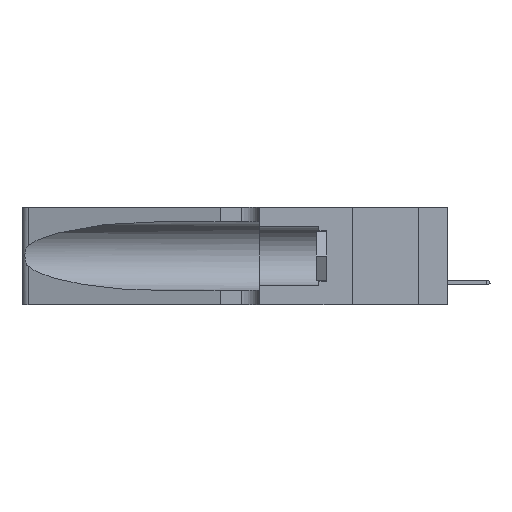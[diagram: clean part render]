
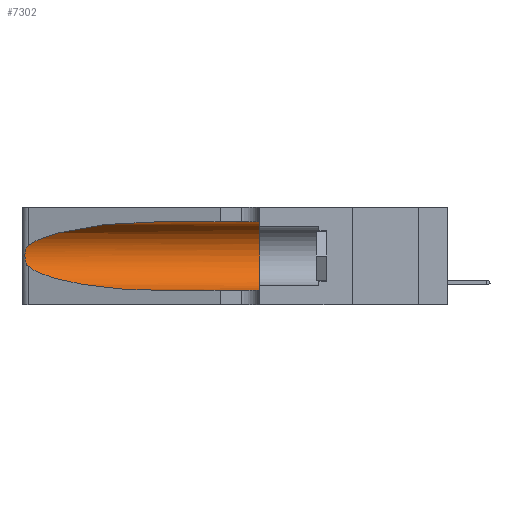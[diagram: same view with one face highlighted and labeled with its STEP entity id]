
A CAD part, left-side view. The second image highlights one B-rep face of the part: STEP entity #7302.
In plain terms, the highlighted cylindrical face has radius 3.308 mm (diameter 6.617 mm), a partial arc.
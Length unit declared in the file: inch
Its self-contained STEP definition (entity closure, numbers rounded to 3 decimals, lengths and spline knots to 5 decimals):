
#775 = CARTESIAN_POINT ( 'NONE',  ( 0.26075, 1.23896, 0.19203 ) ) ;
#2974 = CARTESIAN_POINT ( 'NONE',  ( 0.25639, 1.23184, 0.21858 ) ) ;
#3128 = CARTESIAN_POINT ( 'NONE',  ( 0.25487, 1.22718, 0.22369 ) ) ;
#3421 = CARTESIAN_POINT ( 'NONE',  ( 0.18966, 0.96281, 0.31525 ) ) ;
#3547 = DIRECTION ( 'NONE',  ( 0., 1., 0. ) ) ;
#3717 = CARTESIAN_POINT ( 'NONE',  ( 0.25487, 1.22718, 0.14631 ) ) ;
#3810 = CARTESIAN_POINT ( 'NONE',  ( 0.25487, 1.22718, 0.22369 ) ) ;
#4111 = CARTESIAN_POINT ( 'NONE',  ( 0.2373, 1.15595, 0.08982 ) ) ;
#6169 = CARTESIAN_POINT ( 'NONE',  ( 0.26017, 1.23833, 0.17102 ) ) ;
#6350 = VERTEX_POINT ( 'NONE', #21844 ) ;
#6924 = CARTESIAN_POINT ( 'NONE',  ( 0.25487, 1.22718, 0.14631 ) ) ;
#7302 = ADVANCED_FACE ( 'NONE', ( #29287 ), #10750, .F. ) ;
#8679 = AXIS2_PLACEMENT_3D ( 'NONE', #15345, #21358, #27073 ) ;
#8754 = CARTESIAN_POINT ( 'NONE',  ( 0.25854, 1.2359, 0.20912 ) ) ;
#8937 = EDGE_LOOP ( 'NONE', ( #24188, #16238, #22249, #30770, #29146, #13400 ) ) ;
#9082 = CARTESIAN_POINT ( 'NONE',  ( 0.1305, 0.35, 0.185 ) ) ;
#9935 = VERTEX_POINT ( 'NONE', #6924 ) ;
#10750 = CYLINDRICAL_SURFACE ( 'NONE', #8679, 0.13025 ) ;
#11590 = CARTESIAN_POINT ( 'NONE',  ( 0.25555, 1.22993, 0.14849 ) ) ;
#12124 = VECTOR ( 'NONE', #12397, 39.37008 ) ;
#12397 = DIRECTION ( 'NONE',  ( 0., -1., 0. ) ) ;
#13019 = LINE ( 'NONE', #28895, #12124 ) ;
#13400 = ORIENTED_EDGE ( 'NONE', *, *, #24748, .F. ) ;
#14206 = AXIS2_PLACEMENT_3D ( 'NONE', #9082, #3547, #26107 ) ;
#15270 = CARTESIAN_POINT ( 'NONE',  ( 0.1305, 1.61858, 0.05475 ) ) ;
#15345 = CARTESIAN_POINT ( 'NONE',  ( 0.1305, 1.61858, 0.185 ) ) ;
#15560 = CARTESIAN_POINT ( 'NONE',  ( 0.25487, 1.22718, 0.14631 ) ) ;
#16238 = ORIENTED_EDGE ( 'NONE', *, *, #34376, .T. ) ;
#16996 = CARTESIAN_POINT ( 'NONE',  ( 0.25555, 1.22994, 0.2215 ) ) ;
#17118 = VECTOR ( 'NONE', #34750, 39.37008 ) ;
#17711 = CARTESIAN_POINT ( 'NONE',  ( 0.1305, 0.72297, 0.31525 ) ) ;
#18938 = LINE ( 'NONE', #15270, #17118 ) ;
#19024 = VERTEX_POINT ( 'NONE', #30480 ) ;
#20047 = CARTESIAN_POINT ( 'NONE',  ( 0.25856, 1.23593, 0.16098 ) ) ;
#20294 = CARTESIAN_POINT ( 'NONE',  ( 0.26075, 1.23896, 0.178 ) ) ;
#20326 = EDGE_CURVE ( 'NONE', #29961, #6350, #18938, .T. ) ;
#20816 = CARTESIAN_POINT ( 'NONE',  ( 0.18966, 0.96281, 0.05475 ) ) ;
#21358 = DIRECTION ( 'NONE',  ( 0., -1., 0. ) ) ;
#21844 = CARTESIAN_POINT ( 'NONE',  ( 0.1305, 0.35, 0.05475 ) ) ;
#22249 = ORIENTED_EDGE ( 'NONE', *, *, #34624, .T. ) ;
#22451 = B_SPLINE_CURVE_WITH_KNOTS ( 'NONE', 3,
 ( #22461, #16996, #2974, #25640, #8754, #33553, #775, #20294, #6169, #20047, #31317, #34254, #11590, #3717 ),
 .UNSPECIFIED., .F., .F.,
 ( 4, 2, 2, 2, 2, 2, 4 ),
 ( 0., 0.00027, 0.00053, 0.00107, 0.0016, 0.00187, 0.00214 ),
 .UNSPECIFIED. ) ;
#22461 = CARTESIAN_POINT ( 'NONE',  ( 0.25487, 1.22718, 0.22369 ) ) ;
#23833 = CARTESIAN_POINT ( 'NONE',  ( 0.1305, 0.72297, 0.05475 ) ) ;
#24188 = ORIENTED_EDGE ( 'NONE', *, *, #32831, .T. ) ;
#24748 = EDGE_CURVE ( 'NONE', #26904, #19024, #13019, .T. ) ;
#25640 = CARTESIAN_POINT ( 'NONE',  ( 0.25787, 1.23484, 0.2124 ) ) ;
#26107 = DIRECTION ( 'NONE',  ( 0., 0., 1. ) ) ;
#26265 = CARTESIAN_POINT ( 'NONE',  ( 0.1305, 0.72297, 0.05475 ) ) ;
#26363 = CARTESIAN_POINT ( 'NONE',  ( 0.2373, 1.15595, 0.28018 ) ) ;
#26904 = VERTEX_POINT ( 'NONE', #30628 ) ;
#27073 = DIRECTION ( 'NONE',  ( 0., 0., -1. ) ) ;
#28556 = EDGE_CURVE ( 'NONE', #19024, #6350, #29960, .T. ) ;
#28895 = CARTESIAN_POINT ( 'NONE',  ( 0.1305, 1.61858, 0.31525 ) ) ;
#29146 = ORIENTED_EDGE ( 'NONE', *, *, #28556, .F. ) ;
#29287 = FACE_OUTER_BOUND ( 'NONE', #8937, .T. ) ;
#29960 = CIRCLE ( 'NONE', #14206, 0.13025 ) ;
#29961 = VERTEX_POINT ( 'NONE', #26265 ) ;
#30480 = CARTESIAN_POINT ( 'NONE',  ( 0.1305, 0.35, 0.31525 ) ) ;
#30628 = CARTESIAN_POINT ( 'NONE',  ( 0.1305, 0.72297, 0.31525 ) ) ;
#30770 = ORIENTED_EDGE ( 'NONE', *, *, #20326, .T. ) ;
#31317 = CARTESIAN_POINT ( 'NONE',  ( 0.25789, 1.23486, 0.15765 ) ) ;
#32831 = EDGE_CURVE ( 'NONE', #26904, #33304, #35572, .T. ) ;
#32871 =( BOUNDED_CURVE ( )  B_SPLINE_CURVE ( 3, ( #15560, #4111, #20816, #23833 ),
 .UNSPECIFIED., .F., .T. ) 
 B_SPLINE_CURVE_WITH_KNOTS ( ( 4, 4 ),
 ( 3.44316, 4.71239 ),
 .UNSPECIFIED. ) 
 CURVE ( )  GEOMETRIC_REPRESENTATION_ITEM ( )  RATIONAL_B_SPLINE_CURVE ( ( 1., 0.87, 0.87, 1. ) ) 
 REPRESENTATION_ITEM ( '' )  );
#33304 = VERTEX_POINT ( 'NONE', #3128 ) ;
#33553 = CARTESIAN_POINT ( 'NONE',  ( 0.26018, 1.23835, 0.19895 ) ) ;
#34254 = CARTESIAN_POINT ( 'NONE',  ( 0.25639, 1.23186, 0.15144 ) ) ;
#34376 = EDGE_CURVE ( 'NONE', #33304, #9935, #22451, .T. ) ;
#34624 = EDGE_CURVE ( 'NONE', #9935, #29961, #32871, .T. ) ;
#34750 = DIRECTION ( 'NONE',  ( 0., -1., 0. ) ) ;
#35572 =( BOUNDED_CURVE ( )  B_SPLINE_CURVE ( 3, ( #17711, #3421, #26363, #3810 ),
 .UNSPECIFIED., .F., .F. ) 
 B_SPLINE_CURVE_WITH_KNOTS ( ( 4, 4 ),
 ( 1.5708, 2.84003 ),
 .UNSPECIFIED. ) 
 CURVE ( )  GEOMETRIC_REPRESENTATION_ITEM ( )  RATIONAL_B_SPLINE_CURVE ( ( 1., 0.87, 0.87, 1. ) ) 
 REPRESENTATION_ITEM ( '' )  );
